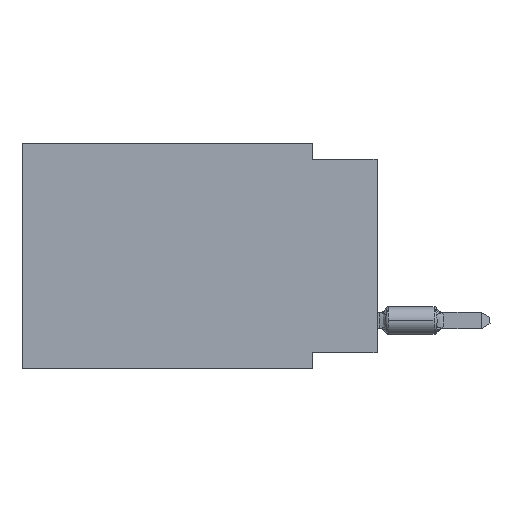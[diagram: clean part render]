
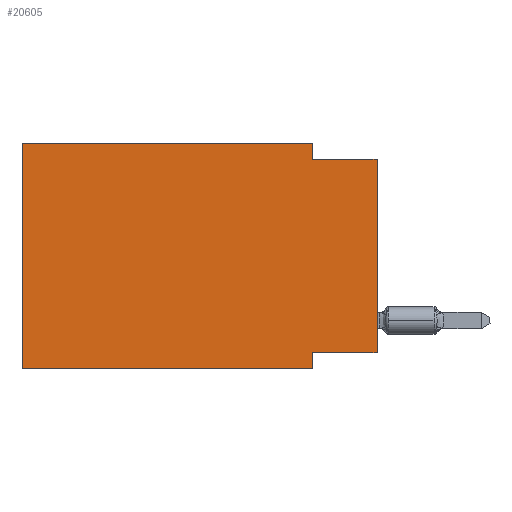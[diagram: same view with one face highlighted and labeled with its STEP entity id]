
A CAD part, left-side view. The second image highlights one B-rep face of the part: STEP entity #20605.
In plain terms, the highlighted planar face has unit normal (-1, 0, 0).
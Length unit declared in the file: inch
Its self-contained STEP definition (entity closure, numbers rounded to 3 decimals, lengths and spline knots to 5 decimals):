
#69 = DIRECTION ( 'NONE',  ( 1., 0., 0. ) ) ;
#232 = CARTESIAN_POINT ( 'NONE',  ( 0., 0.1, 0. ) ) ;
#774 = CARTESIAN_POINT ( 'NONE',  ( 0., 0.55, 0. ) ) ;
#952 = EDGE_CURVE ( 'NONE', #7150, #2649, #2518, .T. ) ;
#997 = VERTEX_POINT ( 'NONE', #5872 ) ;
#1042 = EDGE_CURVE ( 'NONE', #9214, #9531, #13368, .T. ) ;
#1232 = CARTESIAN_POINT ( 'NONE',  ( 0., 0.1, -0.35 ) ) ;
#1287 = VECTOR ( 'NONE', #8544, 39.37008 ) ;
#1463 = ORIENTED_EDGE ( 'NONE', *, *, #8388, .F. ) ;
#2074 = CARTESIAN_POINT ( 'NONE',  ( 0., 0., -0.325 ) ) ;
#2518 = LINE ( 'NONE', #774, #19099 ) ;
#2649 = VERTEX_POINT ( 'NONE', #232 ) ;
#3219 = LINE ( 'NONE', #19067, #20320 ) ;
#3285 = LINE ( 'NONE', #18840, #18854 ) ;
#3523 = CARTESIAN_POINT ( 'NONE',  ( 0., 0., -0.025 ) ) ;
#3823 = AXIS2_PLACEMENT_3D ( 'NONE', #17747, #69, #11393 ) ;
#4349 = LINE ( 'NONE', #2074, #11923 ) ;
#5280 = CARTESIAN_POINT ( 'NONE',  ( 0., 0., -0.025 ) ) ;
#5872 = CARTESIAN_POINT ( 'NONE',  ( 0., 0.1, -0.025 ) ) ;
#5924 = VERTEX_POINT ( 'NONE', #17535 ) ;
#6309 = DIRECTION ( 'NONE',  ( 0., 0., 1. ) ) ;
#6783 = CARTESIAN_POINT ( 'NONE',  ( 0., 0.55, 0. ) ) ;
#7138 = EDGE_LOOP ( 'NONE', ( #20798, #1463, #15423, #9130, #15540, #9164, #18192, #16999 ) ) ;
#7150 = VERTEX_POINT ( 'NONE', #6783 ) ;
#7638 = DIRECTION ( 'NONE',  ( 0., 0., 1. ) ) ;
#8351 = VERTEX_POINT ( 'NONE', #3523 ) ;
#8388 = EDGE_CURVE ( 'NONE', #997, #8351, #9887, .T. ) ;
#8544 = DIRECTION ( 'NONE',  ( 0., -1., 0. ) ) ;
#9130 = ORIENTED_EDGE ( 'NONE', *, *, #952, .F. ) ;
#9164 = ORIENTED_EDGE ( 'NONE', *, *, #1042, .T. ) ;
#9214 = VERTEX_POINT ( 'NONE', #13243 ) ;
#9503 = VECTOR ( 'NONE', #14781, 39.37008 ) ;
#9531 = VERTEX_POINT ( 'NONE', #1232 ) ;
#9887 = LINE ( 'NONE', #5280, #1287 ) ;
#10901 = DIRECTION ( 'NONE',  ( 0., -1., 0. ) ) ;
#11150 = CARTESIAN_POINT ( 'NONE',  ( 0., 0.1, -0.35 ) ) ;
#11393 = DIRECTION ( 'NONE',  ( 0., 0., -1. ) ) ;
#11923 = VECTOR ( 'NONE', #18190, 39.37008 ) ;
#12145 = EDGE_CURVE ( 'NONE', #2649, #997, #14282, .T. ) ;
#12384 = VECTOR ( 'NONE', #10901, 39.37008 ) ;
#12451 = CARTESIAN_POINT ( 'NONE',  ( 0., 0.55, -0.35 ) ) ;
#12949 = PLANE ( 'NONE',  #3823 ) ;
#13243 = CARTESIAN_POINT ( 'NONE',  ( 0., 0.55, -0.35 ) ) ;
#13368 = LINE ( 'NONE', #12451, #12384 ) ;
#13697 = DIRECTION ( 'NONE',  ( 0., -1., 0. ) ) ;
#14282 = LINE ( 'NONE', #16389, #9503 ) ;
#14464 = FACE_OUTER_BOUND ( 'NONE', #7138, .T. ) ;
#14781 = DIRECTION ( 'NONE',  ( 0., 0., -1. ) ) ;
#15187 = VERTEX_POINT ( 'NONE', #16520 ) ;
#15208 = EDGE_CURVE ( 'NONE', #15187, #5924, #4349, .T. ) ;
#15423 = ORIENTED_EDGE ( 'NONE', *, *, #12145, .F. ) ;
#15540 = ORIENTED_EDGE ( 'NONE', *, *, #17059, .F. ) ;
#16389 = CARTESIAN_POINT ( 'NONE',  ( 0., 0.1, 0. ) ) ;
#16520 = CARTESIAN_POINT ( 'NONE',  ( 0., 0., -0.325 ) ) ;
#16999 = ORIENTED_EDGE ( 'NONE', *, *, #15208, .F. ) ;
#17059 = EDGE_CURVE ( 'NONE', #9214, #7150, #3285, .T. ) ;
#17535 = CARTESIAN_POINT ( 'NONE',  ( 0., 0.1, -0.325 ) ) ;
#17747 = CARTESIAN_POINT ( 'NONE',  ( 0., 0.55, 0. ) ) ;
#17791 = EDGE_CURVE ( 'NONE', #5924, #9531, #18582, .T. ) ;
#18082 = VECTOR ( 'NONE', #20721, 39.37008 ) ;
#18190 = DIRECTION ( 'NONE',  ( 0., 1., 0. ) ) ;
#18192 = ORIENTED_EDGE ( 'NONE', *, *, #17791, .F. ) ;
#18371 = EDGE_CURVE ( 'NONE', #15187, #8351, #3219, .T. ) ;
#18582 = LINE ( 'NONE', #11150, #18082 ) ;
#18840 = CARTESIAN_POINT ( 'NONE',  ( 0., 0.55, 0. ) ) ;
#18854 = VECTOR ( 'NONE', #7638, 39.37008 ) ;
#19067 = CARTESIAN_POINT ( 'NONE',  ( 0., 0., 0. ) ) ;
#19099 = VECTOR ( 'NONE', #13697, 39.37008 ) ;
#20320 = VECTOR ( 'NONE', #6309, 39.37008 ) ;
#20605 = ADVANCED_FACE ( 'NONE', ( #14464 ), #12949, .F. ) ;
#20721 = DIRECTION ( 'NONE',  ( 0., 0., -1. ) ) ;
#20798 = ORIENTED_EDGE ( 'NONE', *, *, #18371, .T. ) ;
